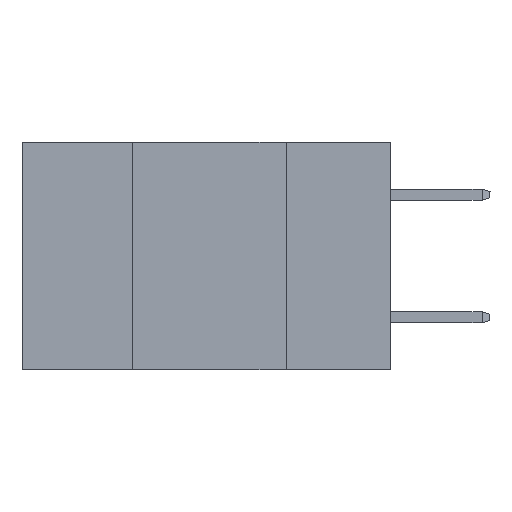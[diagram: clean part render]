
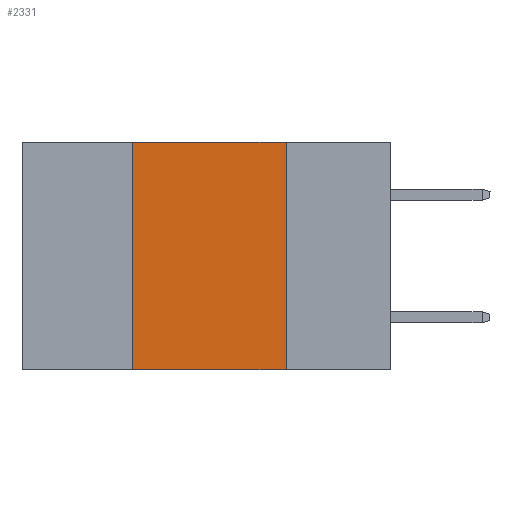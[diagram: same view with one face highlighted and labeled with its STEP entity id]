
A CAD part, left-side view. The second image highlights one B-rep face of the part: STEP entity #2331.
In plain terms, the highlighted planar face has unit normal (-1, 0, 0).
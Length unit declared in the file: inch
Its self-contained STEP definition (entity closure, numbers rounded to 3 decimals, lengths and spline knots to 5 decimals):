
#1701 = CARTESIAN_POINT ( 'NONE',  ( 0., 0.6, 0. ) ) ;
#2331 = ADVANCED_FACE ( 'NONE', ( #14121 ), #17115, .F. ) ;
#3602 = CARTESIAN_POINT ( 'NONE',  ( 0., 0.42, -0.37 ) ) ;
#3604 = LINE ( 'NONE', #33285, #27411 ) ;
#3675 = CARTESIAN_POINT ( 'NONE',  ( 0., 0.6, 0. ) ) ;
#5403 = ORIENTED_EDGE ( 'NONE', *, *, #14342, .T. ) ;
#7124 = CARTESIAN_POINT ( 'NONE',  ( 0., 0.42, 0. ) ) ;
#7476 = DIRECTION ( 'NONE',  ( 0., 0., 1. ) ) ;
#8132 = VERTEX_POINT ( 'NONE', #3602 ) ;
#9303 = VERTEX_POINT ( 'NONE', #32860 ) ;
#10143 = CARTESIAN_POINT ( 'NONE',  ( 0., 0.17, -0.37 ) ) ;
#10747 = CARTESIAN_POINT ( 'NONE',  ( 0., 0.6, -0.37 ) ) ;
#11814 = DIRECTION ( 'NONE',  ( 1., 0., 0. ) ) ;
#12489 = DIRECTION ( 'NONE',  ( 0., -1., 0. ) ) ;
#12750 = ORIENTED_EDGE ( 'NONE', *, *, #16658, .F. ) ;
#12776 = CARTESIAN_POINT ( 'NONE',  ( 0., 0.17, 0. ) ) ;
#14121 = FACE_OUTER_BOUND ( 'NONE', #32699, .T. ) ;
#14342 = EDGE_CURVE ( 'NONE', #8132, #15024, #16909, .T. ) ;
#15024 = VERTEX_POINT ( 'NONE', #10143 ) ;
#15780 = LINE ( 'NONE', #7124, #18969 ) ;
#15810 = VECTOR ( 'NONE', #12489, 39.37008 ) ;
#16658 = EDGE_CURVE ( 'NONE', #9303, #22740, #26255, .T. ) ;
#16909 = LINE ( 'NONE', #10747, #22091 ) ;
#17115 = PLANE ( 'NONE',  #21083 ) ;
#18969 = VECTOR ( 'NONE', #7476, 39.37008 ) ;
#21083 = AXIS2_PLACEMENT_3D ( 'NONE', #3675, #11814, #22582 ) ;
#22091 = VECTOR ( 'NONE', #32281, 39.37008 ) ;
#22102 = ORIENTED_EDGE ( 'NONE', *, *, #33152, .F. ) ;
#22582 = DIRECTION ( 'NONE',  ( 0., 0., -1. ) ) ;
#22740 = VERTEX_POINT ( 'NONE', #12776 ) ;
#25154 = DIRECTION ( 'NONE',  ( 0., 0., -1. ) ) ;
#26255 = LINE ( 'NONE', #1701, #15810 ) ;
#27328 = EDGE_CURVE ( 'NONE', #22740, #15024, #3604, .T. ) ;
#27411 = VECTOR ( 'NONE', #25154, 39.37008 ) ;
#32281 = DIRECTION ( 'NONE',  ( 0., -1., 0. ) ) ;
#32699 = EDGE_LOOP ( 'NONE', ( #33793, #12750, #22102, #5403 ) ) ;
#32860 = CARTESIAN_POINT ( 'NONE',  ( 0., 0.42, 0. ) ) ;
#33152 = EDGE_CURVE ( 'NONE', #8132, #9303, #15780, .T. ) ;
#33285 = CARTESIAN_POINT ( 'NONE',  ( 0., 0.17, 0. ) ) ;
#33793 = ORIENTED_EDGE ( 'NONE', *, *, #27328, .F. ) ;
